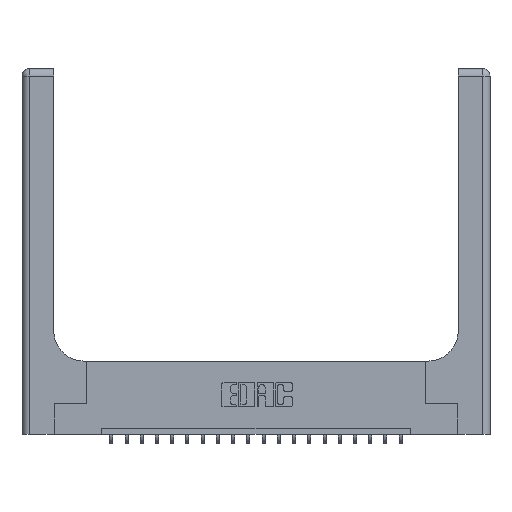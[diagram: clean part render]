
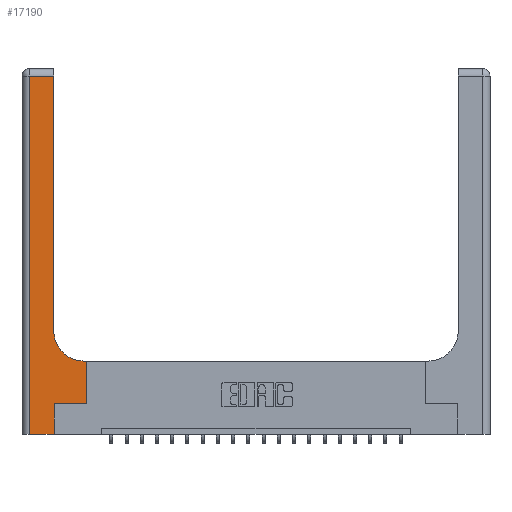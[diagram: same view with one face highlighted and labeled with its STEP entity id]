
A CAD part, top view. The second image highlights one B-rep face of the part: STEP entity #17190.
In plain terms, the highlighted planar face has unit normal (0, 0, 1).
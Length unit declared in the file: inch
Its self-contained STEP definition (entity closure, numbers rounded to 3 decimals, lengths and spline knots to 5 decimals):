
#1935 = CARTESIAN_POINT ( 'NONE',  ( 0., 0., 0.37 ) ) ;
#2107 = CARTESIAN_POINT ( 'NONE',  ( 0.51, 0.6, 0.37 ) ) ;
#2626 = LINE ( 'NONE', #19317, #19078 ) ;
#3287 = VERTEX_POINT ( 'NONE', #2107 ) ;
#3437 = EDGE_LOOP ( 'NONE', ( #15040, #15141, #15247, #15391, #15456, #15543, #15557, #15666, #15688 ) ) ;
#3735 = DIRECTION ( 'NONE',  ( -1., 0., 0. ) ) ;
#3741 = VECTOR ( 'NONE', #14665, 39.37008 ) ;
#4503 = VECTOR ( 'NONE', #9714, 39.37008 ) ;
#5611 = CARTESIAN_POINT ( 'NONE',  ( 0.265, 0., 0.37 ) ) ;
#5888 = DIRECTION ( 'NONE',  ( 0., 1., 0. ) ) ;
#6011 = EDGE_CURVE ( 'NONE', #3287, #7993, #18471, .T. ) ;
#6295 = CARTESIAN_POINT ( 'NONE',  ( 0.265, 0.25, 0.37 ) ) ;
#6814 = EDGE_CURVE ( 'NONE', #7673, #8210, #8719, .T. ) ;
#6884 = CARTESIAN_POINT ( 'NONE',  ( 0.26, 0.85, 0.37 ) ) ;
#7349 = DIRECTION ( 'NONE',  ( 1., 0., 0. ) ) ;
#7673 = VERTEX_POINT ( 'NONE', #13738 ) ;
#7993 = VERTEX_POINT ( 'NONE', #6884 ) ;
#8101 = CARTESIAN_POINT ( 'NONE',  ( 0.528, 0.6, 0.37 ) ) ;
#8133 = CARTESIAN_POINT ( 'NONE',  ( 0.06, 2.94, 0.37 ) ) ;
#8210 = VERTEX_POINT ( 'NONE', #8133 ) ;
#8476 = VERTEX_POINT ( 'NONE', #8748 ) ;
#8481 = PLANE ( 'NONE',  #13846 ) ;
#8718 = FACE_OUTER_BOUND ( 'NONE', #3437, .T. ) ;
#8719 = LINE ( 'NONE', #19245, #4503 ) ;
#8748 = CARTESIAN_POINT ( 'NONE',  ( 0.265, 0., 0.37 ) ) ;
#8992 = CARTESIAN_POINT ( 'NONE',  ( 0.51, 0.85, 0.37 ) ) ;
#9162 = CARTESIAN_POINT ( 'NONE',  ( 0.26, 0.6, 0.37 ) ) ;
#9543 = VECTOR ( 'NONE', #5888, 39.37008 ) ;
#9714 = DIRECTION ( 'NONE',  ( -1., 0., 0. ) ) ;
#10215 = EDGE_CURVE ( 'NONE', #11353, #19126, #17369, .T. ) ;
#10602 = DIRECTION ( 'NONE',  ( 1., 0., 0. ) ) ;
#10773 = DIRECTION ( 'NONE',  ( -1., 0., 0. ) ) ;
#11353 = VERTEX_POINT ( 'NONE', #6295 ) ;
#11491 = EDGE_CURVE ( 'NONE', #8210, #19295, #2626, .T. ) ;
#11531 = VECTOR ( 'NONE', #12015, 39.37008 ) ;
#12015 = DIRECTION ( 'NONE',  ( 0., 1., 0. ) ) ;
#12054 = CARTESIAN_POINT ( 'NONE',  ( 0.06, 0., 0.37 ) ) ;
#12228 = LINE ( 'NONE', #14597, #3741 ) ;
#12983 = VECTOR ( 'NONE', #10773, 39.37008 ) ;
#12996 = DIRECTION ( 'NONE',  ( 0., -1., 0. ) ) ;
#13285 = DIRECTION ( 'NONE',  ( 0., 0., -1. ) ) ;
#13391 = EDGE_CURVE ( 'NONE', #8476, #11353, #15774, .T. ) ;
#13511 = EDGE_CURVE ( 'NONE', #19126, #14014, #14278, .T. ) ;
#13738 = CARTESIAN_POINT ( 'NONE',  ( 0.26, 2.94, 0.37 ) ) ;
#13846 = AXIS2_PLACEMENT_3D ( 'NONE', #19613, #13285, #3735 ) ;
#13954 = VECTOR ( 'NONE', #16384, 39.37008 ) ;
#14014 = VERTEX_POINT ( 'NONE', #8101 ) ;
#14278 = LINE ( 'NONE', #18630, #9543 ) ;
#14597 = CARTESIAN_POINT ( 'NONE',  ( 0.26, 3., 0.37 ) ) ;
#14665 = DIRECTION ( 'NONE',  ( 0., 1., 0. ) ) ;
#14909 = AXIS2_PLACEMENT_3D ( 'NONE', #8992, #20127, #10602 ) ;
#15040 = ORIENTED_EDGE ( 'NONE', *, *, #17116, .T. ) ;
#15141 = ORIENTED_EDGE ( 'NONE', *, *, #6814, .T. ) ;
#15247 = ORIENTED_EDGE ( 'NONE', *, *, #11491, .T. ) ;
#15298 = CARTESIAN_POINT ( 'NONE',  ( 0.265, 0.25, 0.37 ) ) ;
#15391 = ORIENTED_EDGE ( 'NONE', *, *, #18319, .T. ) ;
#15456 = ORIENTED_EDGE ( 'NONE', *, *, #13391, .T. ) ;
#15543 = ORIENTED_EDGE ( 'NONE', *, *, #10215, .T. ) ;
#15557 = ORIENTED_EDGE ( 'NONE', *, *, #13511, .T. ) ;
#15666 = ORIENTED_EDGE ( 'NONE', *, *, #17412, .T. ) ;
#15688 = ORIENTED_EDGE ( 'NONE', *, *, #6011, .T. ) ;
#15774 = LINE ( 'NONE', #5611, #11531 ) ;
#16384 = DIRECTION ( 'NONE',  ( 1., 0., 0. ) ) ;
#16884 = VECTOR ( 'NONE', #7349, 39.37008 ) ;
#17111 = CARTESIAN_POINT ( 'NONE',  ( 0.528, 0.25, 0.37 ) ) ;
#17116 = EDGE_CURVE ( 'NONE', #7993, #7673, #12228, .T. ) ;
#17190 = ADVANCED_FACE ( 'NONE', ( #8718 ), #8481, .F. ) ;
#17221 = LINE ( 'NONE', #9162, #12983 ) ;
#17369 = LINE ( 'NONE', #15298, #16884 ) ;
#17412 = EDGE_CURVE ( 'NONE', #14014, #3287, #17221, .T. ) ;
#18319 = EDGE_CURVE ( 'NONE', #19295, #8476, #18683, .T. ) ;
#18471 = CIRCLE ( 'NONE', #14909, 0.25 ) ;
#18630 = CARTESIAN_POINT ( 'NONE',  ( 0.528, 0.25, 0.37 ) ) ;
#18683 = LINE ( 'NONE', #1935, #13954 ) ;
#19078 = VECTOR ( 'NONE', #12996, 39.37008 ) ;
#19126 = VERTEX_POINT ( 'NONE', #17111 ) ;
#19245 = CARTESIAN_POINT ( 'NONE',  ( 0., 2.94, 0.37 ) ) ;
#19295 = VERTEX_POINT ( 'NONE', #12054 ) ;
#19317 = CARTESIAN_POINT ( 'NONE',  ( 0.06, 3., 0.37 ) ) ;
#19613 = CARTESIAN_POINT ( 'NONE',  ( 0., 3., 0.37 ) ) ;
#20127 = DIRECTION ( 'NONE',  ( 0., 0., -1. ) ) ;
